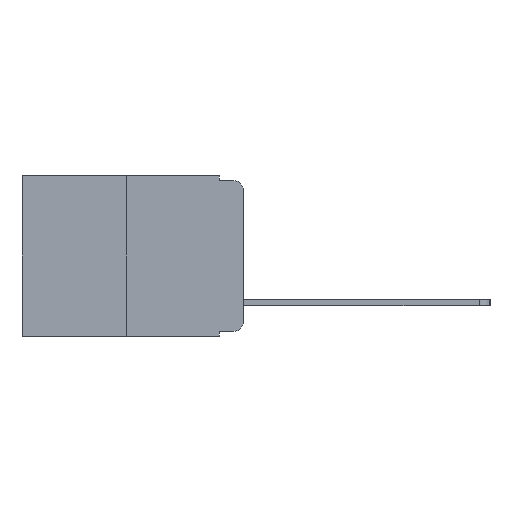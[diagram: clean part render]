
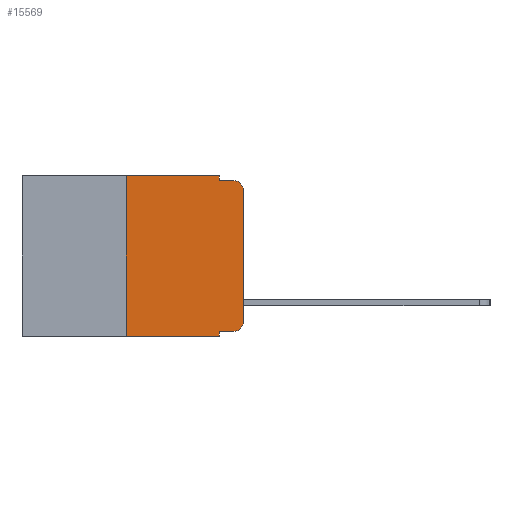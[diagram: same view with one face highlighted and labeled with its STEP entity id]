
A CAD part, left-side view. The second image highlights one B-rep face of the part: STEP entity #15569.
In plain terms, the highlighted planar face has unit normal (-1, 0, 0).
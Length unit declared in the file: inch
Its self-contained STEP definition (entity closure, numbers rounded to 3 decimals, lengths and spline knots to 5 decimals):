
#891 = CARTESIAN_POINT ( 'NONE',  ( 0., 0.02, -0.313 ) ) ;
#1077 = CARTESIAN_POINT ( 'NONE',  ( 0., 0.051, 0. ) ) ;
#1299 = CIRCLE ( 'NONE', #15892, 0.02 ) ;
#1427 = EDGE_LOOP ( 'NONE', ( #21613, #3970, #10643, #22331, #11094, #1513, #14832, #23122, #3068, #8934 ) ) ;
#1441 = CARTESIAN_POINT ( 'NONE',  ( 0., 0.02, -0.01 ) ) ;
#1513 = ORIENTED_EDGE ( 'NONE', *, *, #18437, .F. ) ;
#1549 = VERTEX_POINT ( 'NONE', #1441 ) ;
#1875 = EDGE_CURVE ( 'NONE', #5680, #1549, #18966, .T. ) ;
#2211 = AXIS2_PLACEMENT_3D ( 'NONE', #891, #13950, #3039 ) ;
#2504 = EDGE_CURVE ( 'NONE', #18776, #12290, #16119, .T. ) ;
#2803 = VERTEX_POINT ( 'NONE', #19694 ) ;
#2905 = EDGE_CURVE ( 'NONE', #2803, #20205, #15232, .T. ) ;
#3039 = DIRECTION ( 'NONE',  ( 0., 0., -1. ) ) ;
#3068 = ORIENTED_EDGE ( 'NONE', *, *, #15182, .T. ) ;
#3746 = CARTESIAN_POINT ( 'NONE',  ( 0., 0.051, -0.01 ) ) ;
#3970 = ORIENTED_EDGE ( 'NONE', *, *, #23434, .T. ) ;
#4311 = CARTESIAN_POINT ( 'NONE',  ( 0., 0., -0.03 ) ) ;
#5019 = CARTESIAN_POINT ( 'NONE',  ( 0., 0.25, 0. ) ) ;
#5277 = DIRECTION ( 'NONE',  ( 0., -1., 0. ) ) ;
#5424 = EDGE_CURVE ( 'NONE', #20205, #5680, #14588, .T. ) ;
#5604 = CARTESIAN_POINT ( 'NONE',  ( 0., 0.473, 0. ) ) ;
#5680 = VERTEX_POINT ( 'NONE', #3746 ) ;
#6215 = EDGE_CURVE ( 'NONE', #18767, #12290, #8271, .T. ) ;
#6235 = PLANE ( 'NONE',  #20933 ) ;
#7129 = CARTESIAN_POINT ( 'NONE',  ( 0., 0.051, -0.333 ) ) ;
#7800 = CARTESIAN_POINT ( 'NONE',  ( 0., 0.02, -0.03 ) ) ;
#7980 = LINE ( 'NONE', #5019, #17633 ) ;
#8037 = DIRECTION ( 'NONE',  ( 0., 0., -1. ) ) ;
#8271 = LINE ( 'NONE', #1077, #22191 ) ;
#8388 = EDGE_CURVE ( 'NONE', #12358, #21537, #11794, .T. ) ;
#8504 = CARTESIAN_POINT ( 'NONE',  ( 0., 0.051, 0. ) ) ;
#8648 = CARTESIAN_POINT ( 'NONE',  ( 0., 0.051, -0.343 ) ) ;
#8934 = ORIENTED_EDGE ( 'NONE', *, *, #14418, .T. ) ;
#9012 = VECTOR ( 'NONE', #10680, 39.37008 ) ;
#9241 = DIRECTION ( 'NONE',  ( 0., -1., 0. ) ) ;
#9638 = DIRECTION ( 'NONE',  ( 0., 0., -1. ) ) ;
#10643 = ORIENTED_EDGE ( 'NONE', *, *, #1875, .F. ) ;
#10680 = DIRECTION ( 'NONE',  ( 0., -1., 0. ) ) ;
#10712 = VECTOR ( 'NONE', #14120, 39.37008 ) ;
#10977 = CARTESIAN_POINT ( 'NONE',  ( 0., 0.02, -0.333 ) ) ;
#11094 = ORIENTED_EDGE ( 'NONE', *, *, #2905, .F. ) ;
#11794 = LINE ( 'NONE', #19989, #12370 ) ;
#12290 = VERTEX_POINT ( 'NONE', #8648 ) ;
#12358 = VERTEX_POINT ( 'NONE', #23302 ) ;
#12370 = VECTOR ( 'NONE', #21818, 39.37008 ) ;
#13950 = DIRECTION ( 'NONE',  ( -1., 0., 0. ) ) ;
#14120 = DIRECTION ( 'NONE',  ( 0., -1., 0. ) ) ;
#14194 = VECTOR ( 'NONE', #5277, 39.37008 ) ;
#14407 = LINE ( 'NONE', #7129, #9012 ) ;
#14418 = EDGE_CURVE ( 'NONE', #18063, #12358, #23210, .T. ) ;
#14588 = LINE ( 'NONE', #8504, #15149 ) ;
#14832 = ORIENTED_EDGE ( 'NONE', *, *, #2504, .T. ) ;
#15149 = VECTOR ( 'NONE', #19363, 39.37008 ) ;
#15182 = EDGE_CURVE ( 'NONE', #18767, #18063, #14407, .T. ) ;
#15232 = LINE ( 'NONE', #5604, #20055 ) ;
#15569 = ADVANCED_FACE ( 'NONE', ( #16644 ), #6235, .F. ) ;
#15892 = AXIS2_PLACEMENT_3D ( 'NONE', #7800, #20500, #9638 ) ;
#15896 = DIRECTION ( 'NONE',  ( 0., 0., 1. ) ) ;
#16061 = CARTESIAN_POINT ( 'NONE',  ( 0., 0.051, -0.01 ) ) ;
#16119 = LINE ( 'NONE', #23142, #10712 ) ;
#16644 = FACE_OUTER_BOUND ( 'NONE', #1427, .T. ) ;
#16669 = CARTESIAN_POINT ( 'NONE',  ( 0., 0.25, -0.343 ) ) ;
#17633 = VECTOR ( 'NONE', #15896, 39.37008 ) ;
#18063 = VERTEX_POINT ( 'NONE', #10977 ) ;
#18437 = EDGE_CURVE ( 'NONE', #18776, #2803, #7980, .T. ) ;
#18767 = VERTEX_POINT ( 'NONE', #20314 ) ;
#18776 = VERTEX_POINT ( 'NONE', #16669 ) ;
#18878 = DIRECTION ( 'NONE',  ( 1., 0., 0. ) ) ;
#18966 = LINE ( 'NONE', #16061, #14194 ) ;
#19363 = DIRECTION ( 'NONE',  ( 0., 0., -1. ) ) ;
#19694 = CARTESIAN_POINT ( 'NONE',  ( 0., 0.25, 0. ) ) ;
#19989 = CARTESIAN_POINT ( 'NONE',  ( 0., 0., 0. ) ) ;
#20055 = VECTOR ( 'NONE', #9241, 39.37008 ) ;
#20180 = CARTESIAN_POINT ( 'NONE',  ( 0., 0.051, 0. ) ) ;
#20205 = VERTEX_POINT ( 'NONE', #20180 ) ;
#20314 = CARTESIAN_POINT ( 'NONE',  ( 0., 0.051, -0.333 ) ) ;
#20500 = DIRECTION ( 'NONE',  ( -1., 0., 0. ) ) ;
#20640 = CARTESIAN_POINT ( 'NONE',  ( 0., 0.473, 0. ) ) ;
#20933 = AXIS2_PLACEMENT_3D ( 'NONE', #20640, #18878, #8037 ) ;
#21537 = VERTEX_POINT ( 'NONE', #4311 ) ;
#21613 = ORIENTED_EDGE ( 'NONE', *, *, #8388, .T. ) ;
#21818 = DIRECTION ( 'NONE',  ( 0., 0., 1. ) ) ;
#22191 = VECTOR ( 'NONE', #23147, 39.37008 ) ;
#22331 = ORIENTED_EDGE ( 'NONE', *, *, #5424, .F. ) ;
#23122 = ORIENTED_EDGE ( 'NONE', *, *, #6215, .F. ) ;
#23142 = CARTESIAN_POINT ( 'NONE',  ( 0., 0.473, -0.343 ) ) ;
#23147 = DIRECTION ( 'NONE',  ( 0., 0., -1. ) ) ;
#23210 = CIRCLE ( 'NONE', #2211, 0.02 ) ;
#23302 = CARTESIAN_POINT ( 'NONE',  ( 0., 0., -0.313 ) ) ;
#23434 = EDGE_CURVE ( 'NONE', #21537, #1549, #1299, .T. ) ;
